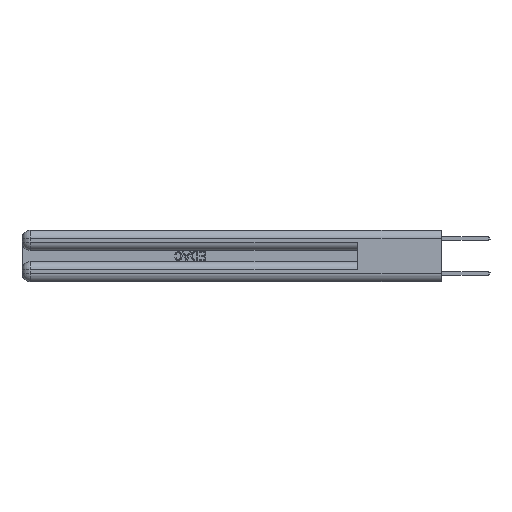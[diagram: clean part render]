
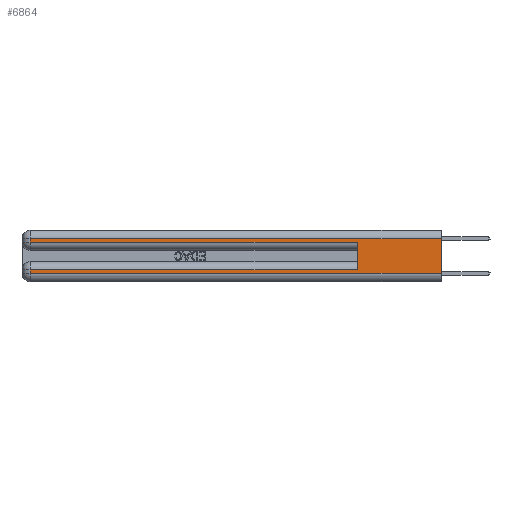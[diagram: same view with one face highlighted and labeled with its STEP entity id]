
A CAD part, left-side view. The second image highlights one B-rep face of the part: STEP entity #6864.
In plain terms, the highlighted planar face has unit normal (-1, 0, 0).
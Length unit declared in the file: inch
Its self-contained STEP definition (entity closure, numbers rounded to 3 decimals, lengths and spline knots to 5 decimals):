
#481 = CARTESIAN_POINT ( 'NONE',  ( 0., 0.6, 0.085 ) ) ;
#672 = FACE_OUTER_BOUND ( 'NONE', #9960, .T. ) ;
#890 = DIRECTION ( 'NONE',  ( 0., -1., 0. ) ) ;
#981 = VECTOR ( 'NONE', #26128, 39.37008 ) ;
#1725 = CARTESIAN_POINT ( 'NONE',  ( 0., 2.94, 0.31 ) ) ;
#1822 = ORIENTED_EDGE ( 'NONE', *, *, #15904, .T. ) ;
#1926 = DIRECTION ( 'NONE',  ( 0., 1., 0. ) ) ;
#2936 = ORIENTED_EDGE ( 'NONE', *, *, #15859, .F. ) ;
#3375 = DIRECTION ( 'NONE',  ( 0., 0., -1. ) ) ;
#4885 = CARTESIAN_POINT ( 'NONE',  ( 0., 2.94, 0.085 ) ) ;
#5332 = LINE ( 'NONE', #32793, #27315 ) ;
#5971 = CARTESIAN_POINT ( 'NONE',  ( 0., 2.94, 0.37 ) ) ;
#6029 = VERTEX_POINT ( 'NONE', #32495 ) ;
#6120 = EDGE_CURVE ( 'NONE', #22393, #31267, #9975, .T. ) ;
#6864 = ADVANCED_FACE ( 'NONE', ( #672 ), #31436, .F. ) ;
#7224 = CARTESIAN_POINT ( 'NONE',  ( 0., 0., 0.31 ) ) ;
#9036 = EDGE_CURVE ( 'NONE', #10383, #33030, #29688, .T. ) ;
#9115 = DIRECTION ( 'NONE',  ( 0., -1., 0. ) ) ;
#9211 = EDGE_CURVE ( 'NONE', #10383, #32129, #5332, .T. ) ;
#9324 = VECTOR ( 'NONE', #890, 39.37008 ) ;
#9960 = EDGE_LOOP ( 'NONE', ( #2936, #26741, #13139, #26293, #11677, #19464, #1822, #12037 ) ) ;
#9975 = LINE ( 'NONE', #7224, #11113 ) ;
#10383 = VERTEX_POINT ( 'NONE', #481 ) ;
#10461 = EDGE_CURVE ( 'NONE', #31267, #24312, #14966, .T. ) ;
#11113 = VECTOR ( 'NONE', #1926, 39.37008 ) ;
#11608 = VECTOR ( 'NONE', #3375, 39.37008 ) ;
#11677 = ORIENTED_EDGE ( 'NONE', *, *, #9036, .F. ) ;
#11970 = LINE ( 'NONE', #12331, #11608 ) ;
#12037 = ORIENTED_EDGE ( 'NONE', *, *, #14878, .T. ) ;
#12331 = CARTESIAN_POINT ( 'NONE',  ( 0., 2.94, 0.37 ) ) ;
#13139 = ORIENTED_EDGE ( 'NONE', *, *, #10461, .T. ) ;
#13567 = CARTESIAN_POINT ( 'NONE',  ( 0., 0., 0.06 ) ) ;
#14693 = AXIS2_PLACEMENT_3D ( 'NONE', #16700, #24934, #17725 ) ;
#14855 = EDGE_CURVE ( 'NONE', #24312, #33030, #25989, .T. ) ;
#14878 = EDGE_CURVE ( 'NONE', #6029, #35019, #23615, .T. ) ;
#14966 = LINE ( 'NONE', #5971, #981 ) ;
#15191 = CARTESIAN_POINT ( 'NONE',  ( 0., 0., 0.285 ) ) ;
#15859 = EDGE_CURVE ( 'NONE', #22393, #35019, #34487, .T. ) ;
#15904 = EDGE_CURVE ( 'NONE', #32129, #6029, #11970, .T. ) ;
#16527 = DIRECTION ( 'NONE',  ( 0., 1., 0. ) ) ;
#16700 = CARTESIAN_POINT ( 'NONE',  ( 0., 0., 0.37 ) ) ;
#17274 = CARTESIAN_POINT ( 'NONE',  ( 0., 2.94, 0.285 ) ) ;
#17725 = DIRECTION ( 'NONE',  ( 0., 0., -1. ) ) ;
#18186 = CARTESIAN_POINT ( 'NONE',  ( 0., 0.6, 0.145 ) ) ;
#18682 = VECTOR ( 'NONE', #31375, 39.37008 ) ;
#19464 = ORIENTED_EDGE ( 'NONE', *, *, #9211, .T. ) ;
#22393 = VERTEX_POINT ( 'NONE', #28963 ) ;
#23615 = LINE ( 'NONE', #23794, #9324 ) ;
#23794 = CARTESIAN_POINT ( 'NONE',  ( 0., 0., 0.06 ) ) ;
#24312 = VERTEX_POINT ( 'NONE', #17274 ) ;
#24934 = DIRECTION ( 'NONE',  ( 1., 0., 0. ) ) ;
#25989 = LINE ( 'NONE', #15191, #31577 ) ;
#26128 = DIRECTION ( 'NONE',  ( 0., 0., -1. ) ) ;
#26293 = ORIENTED_EDGE ( 'NONE', *, *, #14855, .T. ) ;
#26741 = ORIENTED_EDGE ( 'NONE', *, *, #6120, .T. ) ;
#27315 = VECTOR ( 'NONE', #16527, 39.37008 ) ;
#28484 = VECTOR ( 'NONE', #35189, 39.37008 ) ;
#28963 = CARTESIAN_POINT ( 'NONE',  ( 0., 0., 0.31 ) ) ;
#29520 = CARTESIAN_POINT ( 'NONE',  ( 0., 0.6, 0.285 ) ) ;
#29688 = LINE ( 'NONE', #18186, #28484 ) ;
#31267 = VERTEX_POINT ( 'NONE', #1725 ) ;
#31375 = DIRECTION ( 'NONE',  ( 0., 0., -1. ) ) ;
#31436 = PLANE ( 'NONE',  #14693 ) ;
#31577 = VECTOR ( 'NONE', #9115, 39.37008 ) ;
#31733 = CARTESIAN_POINT ( 'NONE',  ( 0., 0., 0.37 ) ) ;
#32129 = VERTEX_POINT ( 'NONE', #4885 ) ;
#32495 = CARTESIAN_POINT ( 'NONE',  ( 0., 2.94, 0.06 ) ) ;
#32793 = CARTESIAN_POINT ( 'NONE',  ( 0., 0., 0.085 ) ) ;
#33030 = VERTEX_POINT ( 'NONE', #29520 ) ;
#34487 = LINE ( 'NONE', #31733, #18682 ) ;
#35019 = VERTEX_POINT ( 'NONE', #13567 ) ;
#35189 = DIRECTION ( 'NONE',  ( 0., 0., 1. ) ) ;
